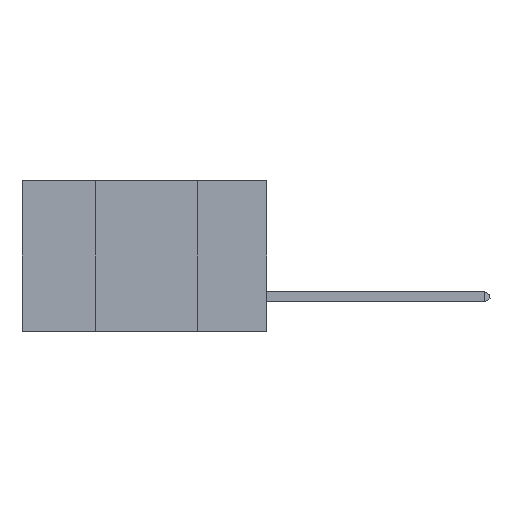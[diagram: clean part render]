
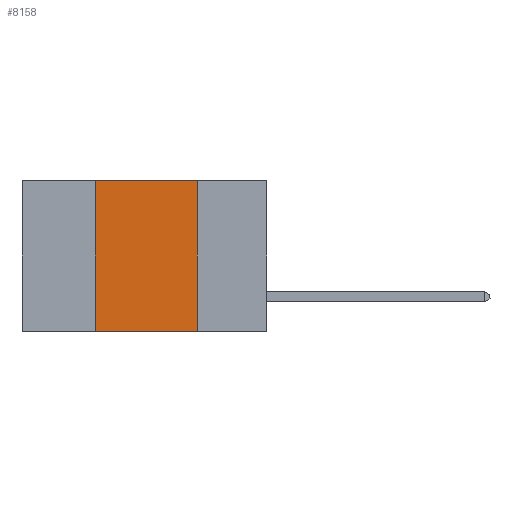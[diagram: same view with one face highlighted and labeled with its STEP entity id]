
A CAD part, left-side view. The second image highlights one B-rep face of the part: STEP entity #8158.
In plain terms, the highlighted planar face has unit normal (-1, 0, 0).
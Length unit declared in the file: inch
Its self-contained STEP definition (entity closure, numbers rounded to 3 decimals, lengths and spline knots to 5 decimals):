
#523 = AXIS2_PLACEMENT_3D ( 'NONE', #5552, #20094, #10475 ) ;
#2243 = CARTESIAN_POINT ( 'NONE',  ( 0., 0.17, 0. ) ) ;
#2508 = CARTESIAN_POINT ( 'NONE',  ( 0., 0.42, -0.37 ) ) ;
#3999 = LINE ( 'NONE', #11288, #12221 ) ;
#4871 = FACE_OUTER_BOUND ( 'NONE', #10819, .T. ) ;
#5044 = CARTESIAN_POINT ( 'NONE',  ( 0., 0.6, -0.37 ) ) ;
#5552 = CARTESIAN_POINT ( 'NONE',  ( 0., 0.6, 0. ) ) ;
#5615 = EDGE_CURVE ( 'NONE', #7104, #15404, #3999, .T. ) ;
#6703 = DIRECTION ( 'NONE',  ( 0., -1., 0. ) ) ;
#6819 = ORIENTED_EDGE ( 'NONE', *, *, #5615, .F. ) ;
#7104 = VERTEX_POINT ( 'NONE', #2243 ) ;
#7951 = VECTOR ( 'NONE', #6703, 39.37008 ) ;
#8158 = ADVANCED_FACE ( 'NONE', ( #4871 ), #8836, .F. ) ;
#8836 = PLANE ( 'NONE',  #523 ) ;
#9774 = CARTESIAN_POINT ( 'NONE',  ( 0., 0.17, -0.37 ) ) ;
#9994 = CARTESIAN_POINT ( 'NONE',  ( 0., 0.42, 0. ) ) ;
#10475 = DIRECTION ( 'NONE',  ( 0., 0., -1. ) ) ;
#10819 = EDGE_LOOP ( 'NONE', ( #6819, #11163, #16001, #20192 ) ) ;
#11163 = ORIENTED_EDGE ( 'NONE', *, *, #12923, .F. ) ;
#11288 = CARTESIAN_POINT ( 'NONE',  ( 0., 0.17, 0. ) ) ;
#12221 = VECTOR ( 'NONE', #12940, 39.37008 ) ;
#12923 = EDGE_CURVE ( 'NONE', #19948, #7104, #16923, .T. ) ;
#12940 = DIRECTION ( 'NONE',  ( 0., 0., -1. ) ) ;
#15014 = CARTESIAN_POINT ( 'NONE',  ( 0., 0.42, 0. ) ) ;
#15404 = VERTEX_POINT ( 'NONE', #9774 ) ;
#15470 = EDGE_CURVE ( 'NONE', #20206, #15404, #20792, .T. ) ;
#15912 = VECTOR ( 'NONE', #19477, 39.37008 ) ;
#16001 = ORIENTED_EDGE ( 'NONE', *, *, #17607, .F. ) ;
#16377 = CARTESIAN_POINT ( 'NONE',  ( 0., 0.6, 0. ) ) ;
#16509 = LINE ( 'NONE', #15014, #19706 ) ;
#16923 = LINE ( 'NONE', #16377, #15912 ) ;
#17607 = EDGE_CURVE ( 'NONE', #20206, #19948, #16509, .T. ) ;
#18149 = DIRECTION ( 'NONE',  ( 0., 0., 1. ) ) ;
#19477 = DIRECTION ( 'NONE',  ( 0., -1., 0. ) ) ;
#19706 = VECTOR ( 'NONE', #18149, 39.37008 ) ;
#19948 = VERTEX_POINT ( 'NONE', #9994 ) ;
#20094 = DIRECTION ( 'NONE',  ( 1., 0., 0. ) ) ;
#20192 = ORIENTED_EDGE ( 'NONE', *, *, #15470, .T. ) ;
#20206 = VERTEX_POINT ( 'NONE', #2508 ) ;
#20792 = LINE ( 'NONE', #5044, #7951 ) ;
